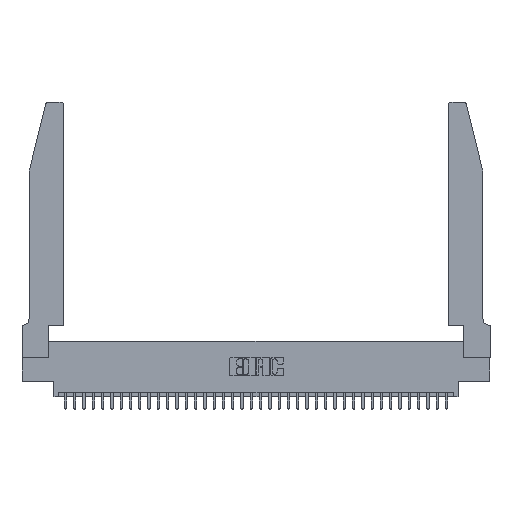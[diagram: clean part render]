
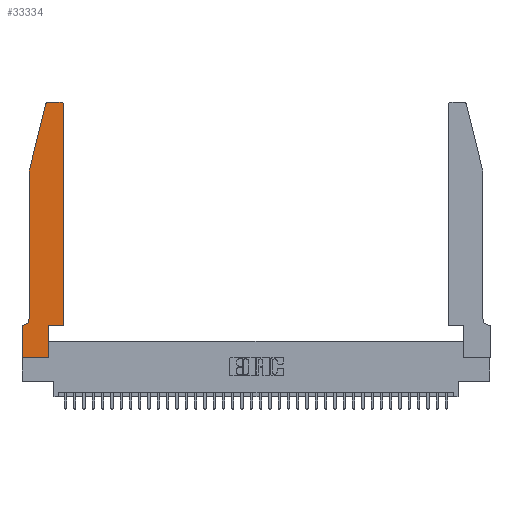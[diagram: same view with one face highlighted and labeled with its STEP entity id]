
A CAD part, top view. The second image highlights one B-rep face of the part: STEP entity #33334.
In plain terms, the highlighted planar face has unit normal (0, 0, 1).
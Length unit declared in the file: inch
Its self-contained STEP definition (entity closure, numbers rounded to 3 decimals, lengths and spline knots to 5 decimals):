
#61 = DIRECTION ( 'NONE',  ( -1., 0., 0. ) ) ;
#179 = VECTOR ( 'NONE', #22638, 39.37008 ) ;
#342 = VERTEX_POINT ( 'NONE', #11326 ) ;
#608 = CARTESIAN_POINT ( 'NONE',  ( 0.4505, 0.35, 0.37 ) ) ;
#827 = EDGE_CURVE ( 'NONE', #33998, #20511, #22686, .T. ) ;
#1833 = LINE ( 'NONE', #24779, #25366 ) ;
#2784 = PLANE ( 'NONE',  #20715 ) ;
#3119 = CARTESIAN_POINT ( 'NONE',  ( 0.0755, 0.42, 0.37 ) ) ;
#3518 = AXIS2_PLACEMENT_3D ( 'NONE', #35172, #17894, #61 ) ;
#3612 = CARTESIAN_POINT ( 'NONE',  ( 0.2865, 0.35, 0.37 ) ) ;
#4051 = CARTESIAN_POINT ( 'NONE',  ( 0.0055, 0.35, 0.37 ) ) ;
#4180 = ORIENTED_EDGE ( 'NONE', *, *, #5195, .T. ) ;
#4933 = LINE ( 'NONE', #11831, #35019 ) ;
#5195 = EDGE_CURVE ( 'NONE', #30557, #6031, #23819, .T. ) ;
#5698 = ORIENTED_EDGE ( 'NONE', *, *, #25049, .T. ) ;
#6031 = VERTEX_POINT ( 'NONE', #3119 ) ;
#6049 = VECTOR ( 'NONE', #19954, 39.37008 ) ;
#6081 = CARTESIAN_POINT ( 'NONE',  ( 0.0755, 2., 0.37 ) ) ;
#6291 = EDGE_CURVE ( 'NONE', #6031, #23038, #25965, .T. ) ;
#6906 = VERTEX_POINT ( 'NONE', #20652 ) ;
#8167 = CARTESIAN_POINT ( 'NONE',  ( 0., 0., 0.37 ) ) ;
#8796 = CARTESIAN_POINT ( 'NONE',  ( 0., 0.35, 0.37 ) ) ;
#9027 = CARTESIAN_POINT ( 'NONE',  ( 0.0755, 2., 0.37 ) ) ;
#9290 = ORIENTED_EDGE ( 'NONE', *, *, #32398, .T. ) ;
#9763 = EDGE_LOOP ( 'NONE', ( #11172, #14357, #9290, #4180, #29394, #21267, #33027, #13490, #30781, #19496, #5698, #37752 ) ) ;
#10698 = FACE_OUTER_BOUND ( 'NONE', #9763, .T. ) ;
#11083 = CARTESIAN_POINT ( 'NONE',  ( 0.2605, 2.75, 0.37 ) ) ;
#11172 = ORIENTED_EDGE ( 'NONE', *, *, #16018, .T. ) ;
#11326 = CARTESIAN_POINT ( 'NONE',  ( 0.4505, 2.72, 0.37 ) ) ;
#11356 = LINE ( 'NONE', #31672, #26002 ) ;
#11743 = DIRECTION ( 'NONE',  ( 1., 0., 0. ) ) ;
#11831 = CARTESIAN_POINT ( 'NONE',  ( 0.4505, 0.35, 0.37 ) ) ;
#13327 = LINE ( 'NONE', #9027, #21133 ) ;
#13490 = ORIENTED_EDGE ( 'NONE', *, *, #32637, .T. ) ;
#13861 = LINE ( 'NONE', #11083, #6049 ) ;
#14357 = ORIENTED_EDGE ( 'NONE', *, *, #18229, .T. ) ;
#14770 = DIRECTION ( 'NONE',  ( 0., 0., 1. ) ) ;
#15065 = DIRECTION ( 'NONE',  ( 0., -1., 0. ) ) ;
#15432 = DIRECTION ( 'NONE',  ( 0., 0., 1. ) ) ;
#16018 = EDGE_CURVE ( 'NONE', #18433, #34172, #13861, .T. ) ;
#17894 = DIRECTION ( 'NONE',  ( 0., 0., -1. ) ) ;
#17927 = AXIS2_PLACEMENT_3D ( 'NONE', #32137, #14770, #35016 ) ;
#17932 = VECTOR ( 'NONE', #19050, 39.37008 ) ;
#18022 = LINE ( 'NONE', #24536, #33002 ) ;
#18164 = CARTESIAN_POINT ( 'NONE',  ( 0., 0.35, 0.37 ) ) ;
#18229 = EDGE_CURVE ( 'NONE', #34172, #6906, #25145, .T. ) ;
#18397 = DIRECTION ( 'NONE',  ( 0., 1., 0. ) ) ;
#18433 = VERTEX_POINT ( 'NONE', #21528 ) ;
#19050 = DIRECTION ( 'NONE',  ( 1., 0., 0. ) ) ;
#19496 = ORIENTED_EDGE ( 'NONE', *, *, #30758, .T. ) ;
#19954 = DIRECTION ( 'NONE',  ( -1., 0., 0. ) ) ;
#20144 = EDGE_CURVE ( 'NONE', #342, #18433, #34422, .T. ) ;
#20157 = VERTEX_POINT ( 'NONE', #3612 ) ;
#20511 = VERTEX_POINT ( 'NONE', #8167 ) ;
#20652 = CARTESIAN_POINT ( 'NONE',  ( 0.25487, 2.72718, 0.37 ) ) ;
#20715 = AXIS2_PLACEMENT_3D ( 'NONE', #8796, #29208, #11743 ) ;
#20960 = CARTESIAN_POINT ( 'NONE',  ( 0., 0., 0.37 ) ) ;
#21133 = VECTOR ( 'NONE', #29460, 39.37008 ) ;
#21267 = ORIENTED_EDGE ( 'NONE', *, *, #30713, .T. ) ;
#21528 = CARTESIAN_POINT ( 'NONE',  ( 0.4205, 2.75, 0.37 ) ) ;
#22108 = AXIS2_PLACEMENT_3D ( 'NONE', #32757, #15432, #35641 ) ;
#22638 = DIRECTION ( 'NONE',  ( 0., -1., 0. ) ) ;
#22686 = LINE ( 'NONE', #20960, #28545 ) ;
#23038 = VERTEX_POINT ( 'NONE', #4051 ) ;
#23819 = LINE ( 'NONE', #34194, #179 ) ;
#24536 = CARTESIAN_POINT ( 'NONE',  ( 0.0755, 0.35, 0.37 ) ) ;
#24779 = CARTESIAN_POINT ( 'NONE',  ( 0.4505, 0.35, 0.37 ) ) ;
#25049 = EDGE_CURVE ( 'NONE', #27876, #342, #4933, .T. ) ;
#25145 = CIRCLE ( 'NONE', #17927, 0.03 ) ;
#25366 = VECTOR ( 'NONE', #27688, 39.37008 ) ;
#25965 = CIRCLE ( 'NONE', #3518, 0.07 ) ;
#26002 = VECTOR ( 'NONE', #34571, 39.37008 ) ;
#26032 = CARTESIAN_POINT ( 'NONE',  ( 0.2865, 0., 0.37 ) ) ;
#27425 = DIRECTION ( 'NONE',  ( -1., 0., 0. ) ) ;
#27532 = CARTESIAN_POINT ( 'NONE',  ( 0.284, 2.75, 0.37 ) ) ;
#27593 = EDGE_CURVE ( 'NONE', #35785, #20157, #11356, .T. ) ;
#27688 = DIRECTION ( 'NONE',  ( 1., 0., 0. ) ) ;
#27876 = VERTEX_POINT ( 'NONE', #608 ) ;
#28545 = VECTOR ( 'NONE', #15065, 39.37008 ) ;
#29208 = DIRECTION ( 'NONE',  ( 0., 0., 1. ) ) ;
#29394 = ORIENTED_EDGE ( 'NONE', *, *, #6291, .T. ) ;
#29460 = DIRECTION ( 'NONE',  ( -0.239, -0.971, 0. ) ) ;
#30550 = CARTESIAN_POINT ( 'NONE',  ( 0., 0., 0.37 ) ) ;
#30557 = VERTEX_POINT ( 'NONE', #6081 ) ;
#30713 = EDGE_CURVE ( 'NONE', #23038, #33998, #18022, .T. ) ;
#30758 = EDGE_CURVE ( 'NONE', #20157, #27876, #1833, .T. ) ;
#30781 = ORIENTED_EDGE ( 'NONE', *, *, #27593, .T. ) ;
#31672 = CARTESIAN_POINT ( 'NONE',  ( 0.2865, 0.35, 0.37 ) ) ;
#32137 = CARTESIAN_POINT ( 'NONE',  ( 0.284, 2.72, 0.37 ) ) ;
#32398 = EDGE_CURVE ( 'NONE', #6906, #30557, #13327, .T. ) ;
#32637 = EDGE_CURVE ( 'NONE', #20511, #35785, #33289, .T. ) ;
#32757 = CARTESIAN_POINT ( 'NONE',  ( 0.4205, 2.72, 0.37 ) ) ;
#33002 = VECTOR ( 'NONE', #27425, 39.37008 ) ;
#33027 = ORIENTED_EDGE ( 'NONE', *, *, #827, .T. ) ;
#33289 = LINE ( 'NONE', #30550, #17932 ) ;
#33334 = ADVANCED_FACE ( 'NONE', ( #10698 ), #2784, .T. ) ;
#33998 = VERTEX_POINT ( 'NONE', #18164 ) ;
#34172 = VERTEX_POINT ( 'NONE', #27532 ) ;
#34194 = CARTESIAN_POINT ( 'NONE',  ( 0.0755, 2., 0.37 ) ) ;
#34422 = CIRCLE ( 'NONE', #22108, 0.03 ) ;
#34571 = DIRECTION ( 'NONE',  ( 0., 1., 0. ) ) ;
#35016 = DIRECTION ( 'NONE',  ( 1., 0., 0. ) ) ;
#35019 = VECTOR ( 'NONE', #18397, 39.37008 ) ;
#35172 = CARTESIAN_POINT ( 'NONE',  ( 0.0055, 0.42, 0.37 ) ) ;
#35641 = DIRECTION ( 'NONE',  ( 1., 0., 0. ) ) ;
#35785 = VERTEX_POINT ( 'NONE', #26032 ) ;
#37752 = ORIENTED_EDGE ( 'NONE', *, *, #20144, .T. ) ;
